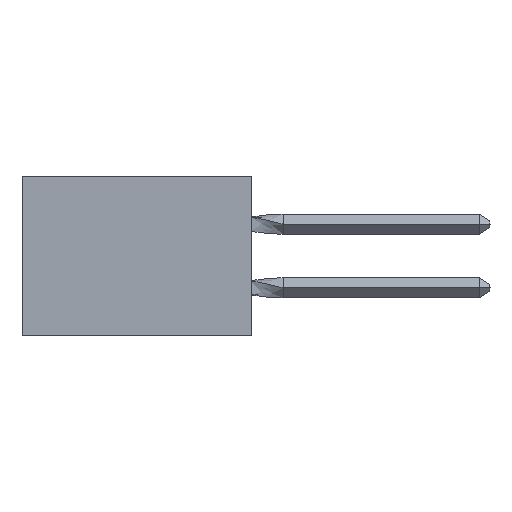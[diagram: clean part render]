
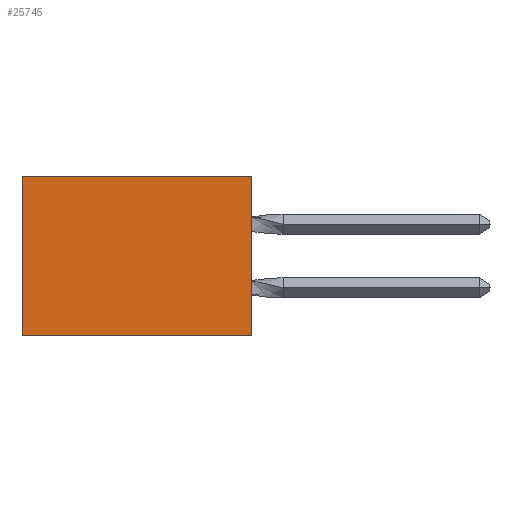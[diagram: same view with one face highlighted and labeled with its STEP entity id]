
A CAD part, left-side view. The second image highlights one B-rep face of the part: STEP entity #25745.
In plain terms, the highlighted planar face has unit normal (-1, 0, 0).
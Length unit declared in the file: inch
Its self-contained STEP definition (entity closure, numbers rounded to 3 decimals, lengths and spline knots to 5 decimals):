
#59 = CARTESIAN_POINT ( 'NONE',  ( 0.305, 0., -0.5 ) ) ;
#1105 = DIRECTION ( 'NONE',  ( 0., 1., 0. ) ) ;
#1380 = VECTOR ( 'NONE', #40815, 39.37008 ) ;
#2545 = EDGE_CURVE ( 'NONE', #37585, #4306, #34145, .T. ) ;
#2593 = EDGE_LOOP ( 'NONE', ( #9173, #38626, #22789, #27785 ) ) ;
#3244 = DIRECTION ( 'NONE',  ( 1., 0., 0. ) ) ;
#3499 = VERTEX_POINT ( 'NONE', #38034 ) ;
#4306 = VERTEX_POINT ( 'NONE', #29965 ) ;
#4477 = CARTESIAN_POINT ( 'NONE',  ( 0.305, 0., 0. ) ) ;
#5446 = EDGE_CURVE ( 'NONE', #37585, #3499, #35807, .T. ) ;
#9173 = ORIENTED_EDGE ( 'NONE', *, *, #39292, .T. ) ;
#9499 = VECTOR ( 'NONE', #25000, 39.37008 ) ;
#9884 = CARTESIAN_POINT ( 'NONE',  ( 0.305, 0., -0.5 ) ) ;
#12239 = CARTESIAN_POINT ( 'NONE',  ( 0.305, 0.72, -0.5 ) ) ;
#13262 = VECTOR ( 'NONE', #1105, 39.37008 ) ;
#14251 = CARTESIAN_POINT ( 'NONE',  ( 0.305, 0.72, -0.5 ) ) ;
#14969 = AXIS2_PLACEMENT_3D ( 'NONE', #59, #3244, #38147 ) ;
#20628 = VECTOR ( 'NONE', #32070, 39.37008 ) ;
#22246 = PLANE ( 'NONE',  #14969 ) ;
#22789 = ORIENTED_EDGE ( 'NONE', *, *, #5446, .F. ) ;
#24564 = LINE ( 'NONE', #9884, #20628 ) ;
#25000 = DIRECTION ( 'NONE',  ( 0., 0., -1. ) ) ;
#25745 = ADVANCED_FACE ( 'NONE', ( #32513 ), #22246, .F. ) ;
#26491 = CARTESIAN_POINT ( 'NONE',  ( 0.305, 0., 0. ) ) ;
#27111 = VERTEX_POINT ( 'NONE', #14251 ) ;
#27785 = ORIENTED_EDGE ( 'NONE', *, *, #2545, .T. ) ;
#29965 = CARTESIAN_POINT ( 'NONE',  ( 0.305, 0.72, 0. ) ) ;
#32070 = DIRECTION ( 'NONE',  ( 0., 1., 0. ) ) ;
#32513 = FACE_OUTER_BOUND ( 'NONE', #2593, .T. ) ;
#34145 = LINE ( 'NONE', #26491, #13262 ) ;
#34254 = CARTESIAN_POINT ( 'NONE',  ( 0.305, 0., -0.5 ) ) ;
#35807 = LINE ( 'NONE', #34254, #9499 ) ;
#37585 = VERTEX_POINT ( 'NONE', #4477 ) ;
#38034 = CARTESIAN_POINT ( 'NONE',  ( 0.305, 0., -0.5 ) ) ;
#38147 = DIRECTION ( 'NONE',  ( 0., 0., -1. ) ) ;
#38626 = ORIENTED_EDGE ( 'NONE', *, *, #38871, .F. ) ;
#38871 = EDGE_CURVE ( 'NONE', #3499, #27111, #24564, .T. ) ;
#39292 = EDGE_CURVE ( 'NONE', #4306, #27111, #40993, .T. ) ;
#40815 = DIRECTION ( 'NONE',  ( 0., 0., -1. ) ) ;
#40993 = LINE ( 'NONE', #12239, #1380 ) ;
